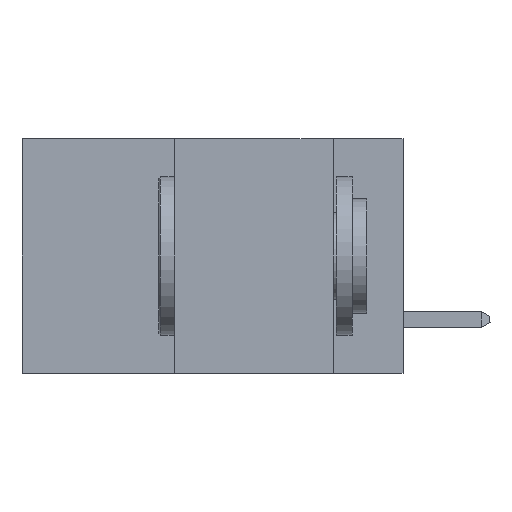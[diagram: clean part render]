
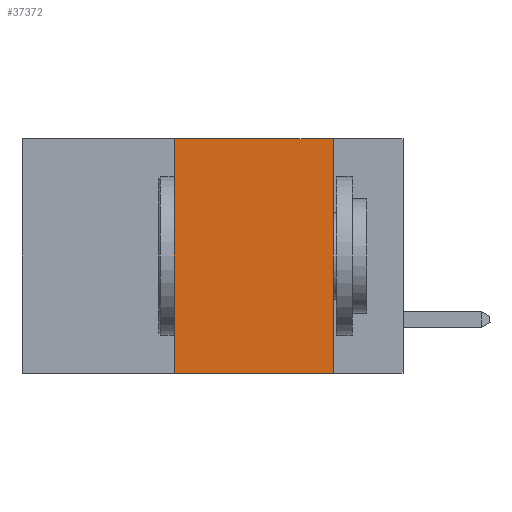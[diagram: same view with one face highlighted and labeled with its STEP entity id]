
A CAD part, left-side view. The second image highlights one B-rep face of the part: STEP entity #37372.
In plain terms, the highlighted planar face has unit normal (-1, 0, 0).
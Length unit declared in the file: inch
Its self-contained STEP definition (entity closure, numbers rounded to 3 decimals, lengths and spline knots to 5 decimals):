
#3968 = DIRECTION ( 'NONE',  ( 1., 0., 0. ) ) ;
#5082 = LINE ( 'NONE', #16451, #21501 ) ;
#6892 = EDGE_CURVE ( 'NONE', #24946, #28128, #39513, .T. ) ;
#8240 = DIRECTION ( 'NONE',  ( 0., -1., 0. ) ) ;
#9414 = AXIS2_PLACEMENT_3D ( 'NONE', #23587, #3968, #26823 ) ;
#9781 = CARTESIAN_POINT ( 'NONE',  ( 0., 0.11, 0. ) ) ;
#12492 = VECTOR ( 'NONE', #30229, 39.37008 ) ;
#14342 = VECTOR ( 'NONE', #36137, 39.37008 ) ;
#14858 = EDGE_CURVE ( 'NONE', #24946, #41895, #5082, .T. ) ;
#16451 = CARTESIAN_POINT ( 'NONE',  ( 0., 0.36, 0. ) ) ;
#18234 = ORIENTED_EDGE ( 'NONE', *, *, #19007, .F. ) ;
#19007 = EDGE_CURVE ( 'NONE', #21562, #28128, #23035, .T. ) ;
#19847 = CARTESIAN_POINT ( 'NONE',  ( 0., 0.11, 0. ) ) ;
#21501 = VECTOR ( 'NONE', #39213, 39.37008 ) ;
#21562 = VERTEX_POINT ( 'NONE', #9781 ) ;
#23035 = LINE ( 'NONE', #19847, #14342 ) ;
#23587 = CARTESIAN_POINT ( 'NONE',  ( 0., 0.6, 0. ) ) ;
#24946 = VERTEX_POINT ( 'NONE', #27746 ) ;
#25572 = FACE_OUTER_BOUND ( 'NONE', #29249, .T. ) ;
#26823 = DIRECTION ( 'NONE',  ( 0., 0., -1. ) ) ;
#27746 = CARTESIAN_POINT ( 'NONE',  ( 0., 0.36, -0.37 ) ) ;
#28128 = VERTEX_POINT ( 'NONE', #31988 ) ;
#29249 = EDGE_LOOP ( 'NONE', ( #18234, #40578, #42130, #37566 ) ) ;
#30229 = DIRECTION ( 'NONE',  ( 0., -1., 0. ) ) ;
#31988 = CARTESIAN_POINT ( 'NONE',  ( 0., 0.11, -0.37 ) ) ;
#36137 = DIRECTION ( 'NONE',  ( 0., 0., -1. ) ) ;
#36273 = EDGE_CURVE ( 'NONE', #41895, #21562, #37891, .T. ) ;
#36729 = CARTESIAN_POINT ( 'NONE',  ( 0., 0.6, -0.37 ) ) ;
#36852 = VECTOR ( 'NONE', #8240, 39.37008 ) ;
#37372 = ADVANCED_FACE ( 'NONE', ( #25572 ), #39783, .F. ) ;
#37443 = CARTESIAN_POINT ( 'NONE',  ( 0., 0.6, 0. ) ) ;
#37566 = ORIENTED_EDGE ( 'NONE', *, *, #6892, .T. ) ;
#37891 = LINE ( 'NONE', #37443, #36852 ) ;
#39213 = DIRECTION ( 'NONE',  ( 0., 0., 1. ) ) ;
#39513 = LINE ( 'NONE', #36729, #12492 ) ;
#39783 = PLANE ( 'NONE',  #9414 ) ;
#40578 = ORIENTED_EDGE ( 'NONE', *, *, #36273, .F. ) ;
#41381 = CARTESIAN_POINT ( 'NONE',  ( 0., 0.36, 0. ) ) ;
#41895 = VERTEX_POINT ( 'NONE', #41381 ) ;
#42130 = ORIENTED_EDGE ( 'NONE', *, *, #14858, .F. ) ;
